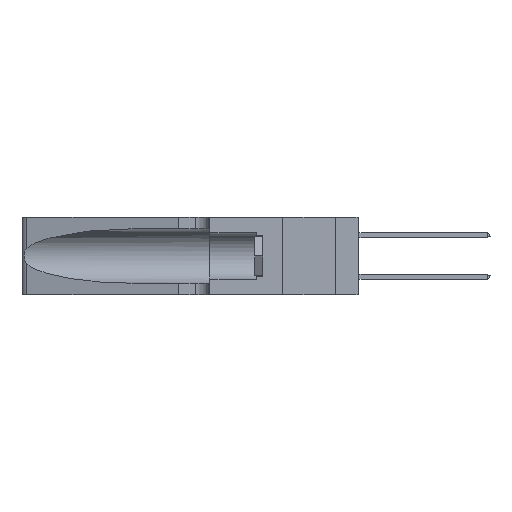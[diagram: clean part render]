
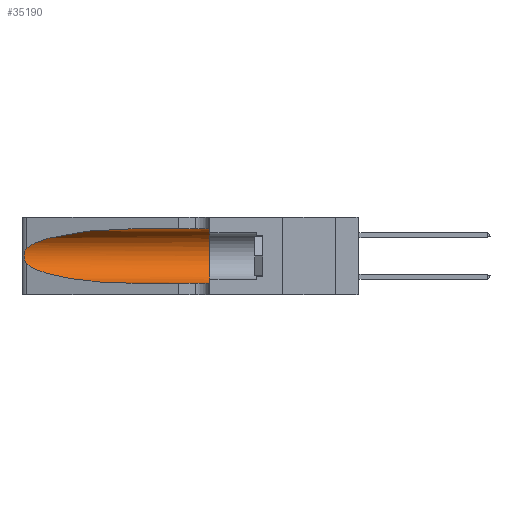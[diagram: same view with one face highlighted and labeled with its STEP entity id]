
A CAD part, left-side view. The second image highlights one B-rep face of the part: STEP entity #35190.
In plain terms, the highlighted cylindrical face has radius 3.308 mm (diameter 6.617 mm), a partial arc.
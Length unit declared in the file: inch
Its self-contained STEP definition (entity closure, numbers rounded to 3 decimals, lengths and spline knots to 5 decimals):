
#202 = ORIENTED_EDGE ( 'NONE', *, *, #16488, .T. ) ;
#416 = VERTEX_POINT ( 'NONE', #31435 ) ;
#916 = CARTESIAN_POINT ( 'NONE',  ( 0.25487, 1.22718, 0.14631 ) ) ;
#1176 = CARTESIAN_POINT ( 'NONE',  ( 0.25856, 1.23593, 0.16098 ) ) ;
#1909 = FACE_OUTER_BOUND ( 'NONE', #28020, .T. ) ;
#2145 = ORIENTED_EDGE ( 'NONE', *, *, #30536, .F. ) ;
#2661 = EDGE_CURVE ( 'NONE', #416, #2742, #40472, .T. ) ;
#2742 = VERTEX_POINT ( 'NONE', #37510 ) ;
#3329 = LINE ( 'NONE', #30950, #21402 ) ;
#3747 =( BOUNDED_CURVE ( )  B_SPLINE_CURVE ( 3, ( #916, #8091, #8241, #33219 ),
 .UNSPECIFIED., .F., .T. ) 
 B_SPLINE_CURVE_WITH_KNOTS ( ( 4, 4 ),
 ( 3.44316, 4.71239 ),
 .UNSPECIFIED. ) 
 CURVE ( )  GEOMETRIC_REPRESENTATION_ITEM ( )  RATIONAL_B_SPLINE_CURVE ( ( 1., 0.87, 0.87, 1. ) ) 
 REPRESENTATION_ITEM ( '' )  );
#4282 = CIRCLE ( 'NONE', #45255, 0.13025 ) ;
#4366 = ORIENTED_EDGE ( 'NONE', *, *, #35026, .F. ) ;
#4756 = CARTESIAN_POINT ( 'NONE',  ( 0.1305, 1.61858, 0.31525 ) ) ;
#4795 = CARTESIAN_POINT ( 'NONE',  ( 0.25639, 1.23186, 0.15144 ) ) ;
#8091 = CARTESIAN_POINT ( 'NONE',  ( 0.2373, 1.15595, 0.08982 ) ) ;
#8241 = CARTESIAN_POINT ( 'NONE',  ( 0.18966, 0.96281, 0.05475 ) ) ;
#8456 = DIRECTION ( 'NONE',  ( 0., -1., 0. ) ) ;
#8495 = CARTESIAN_POINT ( 'NONE',  ( 0.25487, 1.22718, 0.14631 ) ) ;
#8558 = CARTESIAN_POINT ( 'NONE',  ( 0.18966, 0.96281, 0.31525 ) ) ;
#9230 = CARTESIAN_POINT ( 'NONE',  ( 0.1305, 0.35, 0.185 ) ) ;
#9285 = CYLINDRICAL_SURFACE ( 'NONE', #18582, 0.13025 ) ;
#11946 = CARTESIAN_POINT ( 'NONE',  ( 0.25639, 1.23184, 0.21858 ) ) ;
#12024 = CARTESIAN_POINT ( 'NONE',  ( 0.1305, 0.35, 0.31525 ) ) ;
#12612 = CARTESIAN_POINT ( 'NONE',  ( 0.1305, 0.72297, 0.31525 ) ) ;
#12694 = CARTESIAN_POINT ( 'NONE',  ( 0.1305, 1.61858, 0.185 ) ) ;
#12836 = DIRECTION ( 'NONE',  ( 0., 0., 1. ) ) ;
#15562 = CARTESIAN_POINT ( 'NONE',  ( 0.25854, 1.2359, 0.20912 ) ) ;
#15662 =( BOUNDED_CURVE ( )  B_SPLINE_CURVE ( 3, ( #29992, #8558, #19410, #44256 ),
 .UNSPECIFIED., .F., .F. ) 
 B_SPLINE_CURVE_WITH_KNOTS ( ( 4, 4 ),
 ( 1.5708, 2.84003 ),
 .UNSPECIFIED. ) 
 CURVE ( )  GEOMETRIC_REPRESENTATION_ITEM ( )  RATIONAL_B_SPLINE_CURVE ( ( 1., 0.87, 0.87, 1. ) ) 
 REPRESENTATION_ITEM ( '' )  );
#16054 = VECTOR ( 'NONE', #8456, 39.37008 ) ;
#16488 = EDGE_CURVE ( 'NONE', #40130, #416, #15662, .T. ) ;
#17193 = LINE ( 'NONE', #4756, #16054 ) ;
#18582 = AXIS2_PLACEMENT_3D ( 'NONE', #12694, #30633, #23513 ) ;
#19185 = CARTESIAN_POINT ( 'NONE',  ( 0.26075, 1.23896, 0.19203 ) ) ;
#19410 = CARTESIAN_POINT ( 'NONE',  ( 0.2373, 1.15595, 0.28018 ) ) ;
#19445 = ORIENTED_EDGE ( 'NONE', *, *, #2661, .T. ) ;
#20547 = VERTEX_POINT ( 'NONE', #25499 ) ;
#21402 = VECTOR ( 'NONE', #34501, 39.37008 ) ;
#22642 = CARTESIAN_POINT ( 'NONE',  ( 0.25555, 1.22994, 0.2215 ) ) ;
#22807 = CARTESIAN_POINT ( 'NONE',  ( 0.26017, 1.23833, 0.17102 ) ) ;
#23513 = DIRECTION ( 'NONE',  ( 0., 0., -1. ) ) ;
#25499 = CARTESIAN_POINT ( 'NONE',  ( 0.1305, 0.72297, 0.05475 ) ) ;
#26352 = CARTESIAN_POINT ( 'NONE',  ( 0.25789, 1.23486, 0.15765 ) ) ;
#27030 = EDGE_CURVE ( 'NONE', #20547, #39700, #3329, .T. ) ;
#28020 = EDGE_LOOP ( 'NONE', ( #202, #19445, #41665, #45014, #2145, #4366 ) ) ;
#28117 = CARTESIAN_POINT ( 'NONE',  ( 0.1305, 0.35, 0.05475 ) ) ;
#29921 = CARTESIAN_POINT ( 'NONE',  ( 0.25555, 1.22993, 0.14849 ) ) ;
#29992 = CARTESIAN_POINT ( 'NONE',  ( 0.1305, 0.72297, 0.31525 ) ) ;
#30536 = EDGE_CURVE ( 'NONE', #32269, #39700, #4282, .T. ) ;
#30633 = DIRECTION ( 'NONE',  ( 0., -1., 0. ) ) ;
#30950 = CARTESIAN_POINT ( 'NONE',  ( 0.1305, 1.61858, 0.05475 ) ) ;
#31435 = CARTESIAN_POINT ( 'NONE',  ( 0.25487, 1.22718, 0.22369 ) ) ;
#32269 = VERTEX_POINT ( 'NONE', #12024 ) ;
#33153 = CARTESIAN_POINT ( 'NONE',  ( 0.25487, 1.22718, 0.22369 ) ) ;
#33219 = CARTESIAN_POINT ( 'NONE',  ( 0.1305, 0.72297, 0.05475 ) ) ;
#34195 = DIRECTION ( 'NONE',  ( 0., 1., 0. ) ) ;
#34501 = DIRECTION ( 'NONE',  ( 0., -1., 0. ) ) ;
#35026 = EDGE_CURVE ( 'NONE', #40130, #32269, #17193, .T. ) ;
#35190 = ADVANCED_FACE ( 'NONE', ( #1909 ), #9285, .F. ) ;
#36882 = CARTESIAN_POINT ( 'NONE',  ( 0.25787, 1.23484, 0.2124 ) ) ;
#37510 = CARTESIAN_POINT ( 'NONE',  ( 0.25487, 1.22718, 0.14631 ) ) ;
#37614 = EDGE_CURVE ( 'NONE', #2742, #20547, #3747, .T. ) ;
#39700 = VERTEX_POINT ( 'NONE', #28117 ) ;
#40130 = VERTEX_POINT ( 'NONE', #12612 ) ;
#40457 = CARTESIAN_POINT ( 'NONE',  ( 0.26018, 1.23835, 0.19895 ) ) ;
#40472 = B_SPLINE_CURVE_WITH_KNOTS ( 'NONE', 3,
 ( #33153, #22642, #11946, #36882, #15562, #40457, #19185, #44024, #22807, #1176, #26352, #4795, #29921, #8495 ),
 .UNSPECIFIED., .F., .F.,
 ( 4, 2, 2, 2, 2, 2, 4 ),
 ( 0., 0.00027, 0.00053, 0.00107, 0.0016, 0.00187, 0.00214 ),
 .UNSPECIFIED. ) ;
#41665 = ORIENTED_EDGE ( 'NONE', *, *, #37614, .T. ) ;
#44024 = CARTESIAN_POINT ( 'NONE',  ( 0.26075, 1.23896, 0.178 ) ) ;
#44256 = CARTESIAN_POINT ( 'NONE',  ( 0.25487, 1.22718, 0.22369 ) ) ;
#45014 = ORIENTED_EDGE ( 'NONE', *, *, #27030, .T. ) ;
#45255 = AXIS2_PLACEMENT_3D ( 'NONE', #9230, #34195, #12836 ) ;
